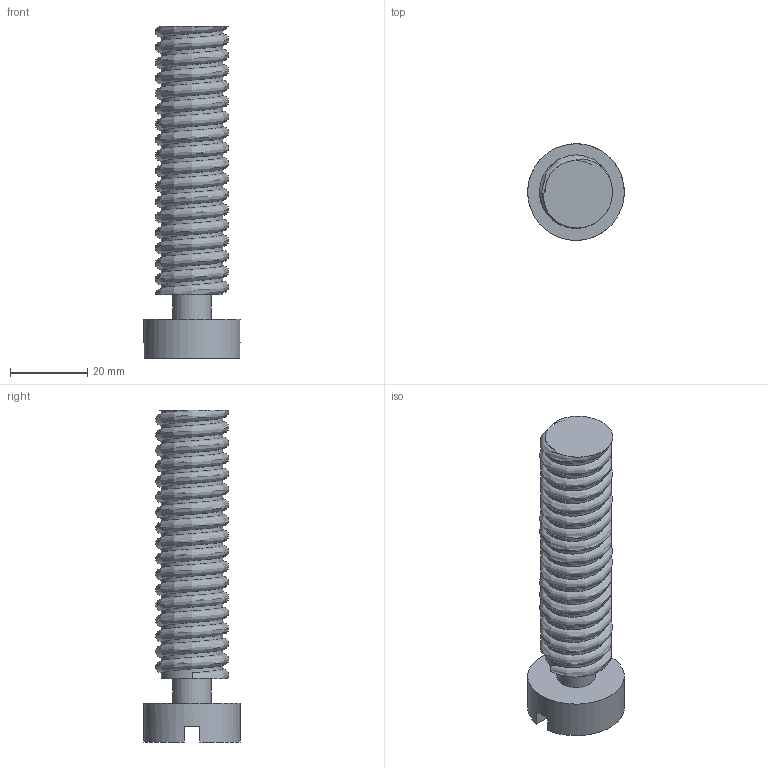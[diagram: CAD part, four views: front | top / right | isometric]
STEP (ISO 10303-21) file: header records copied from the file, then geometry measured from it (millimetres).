
FILE_DESCRIPTION (( 'STEP AP214' ), '1' );
FILE_NAME ('Trellais_Rear_Adjust.step', '2016-04-19T10:44:34', ( 'WarFairy' ), ( '' ), 'SwSTEP 2.0', 'SolidWorks 2015', '' );
FILE_SCHEMA (( 'AUTOMOTIVE_DESIGN' ));
Length unit declared in the file: millimetre
Products named in the file (1): Trellais_Rear_Adjust
Bounding box: 25 x 24.96 x 85.9 mm (x, y, z)
Volume: 22416.8 mm3; surface area: 7967.5 mm2
Topology: 1 solids, 1 shells, 13 faces, 28 edges, 19 vertices
Faces by surface type: plane 9, cylinder 3, bspline 1
Full cylindrical faces by diameter (mm): 10 x1, 25 x1
Entity records: 4352 total; most frequent: CARTESIAN_POINT 4055, DIRECTION 56, ORIENTED_EDGE 48, EDGE_CURVE 24, AXIS2_PLACEMENT_3D 23, VERTEX_POINT 17, EDGE_LOOP 17, FACE_OUTER_BOUND 15
